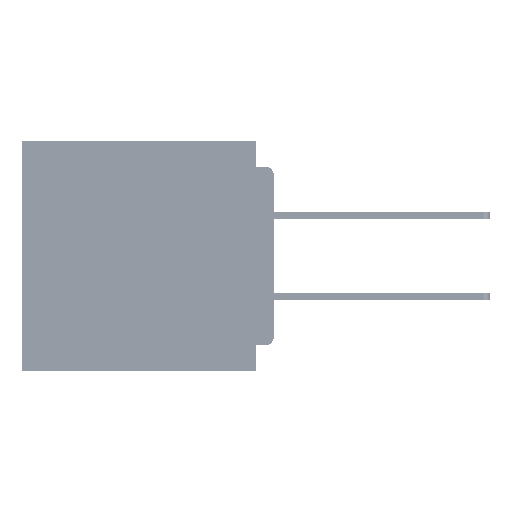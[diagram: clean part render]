
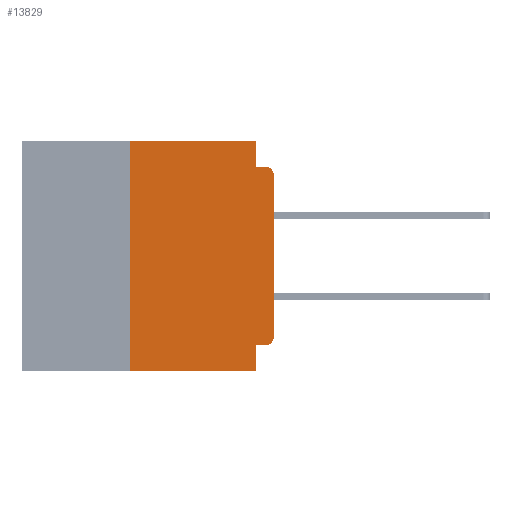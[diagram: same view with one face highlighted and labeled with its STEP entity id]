
A CAD part, left-side view. The second image highlights one B-rep face of the part: STEP entity #13829.
In plain terms, the highlighted planar face has unit normal (-1, 0, 0).
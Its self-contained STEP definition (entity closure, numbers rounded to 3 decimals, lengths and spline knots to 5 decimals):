
#407 = CARTESIAN_POINT ( 'NONE',  ( 0., 0.031, 0. ) ) ;
#1794 = EDGE_CURVE ( 'NONE', #19560, #12595, #44876, .T. ) ;
#2747 = CARTESIAN_POINT ( 'NONE',  ( 0., 0.015, -0.34 ) ) ;
#4199 = CARTESIAN_POINT ( 'NONE',  ( 0., 0.25, -0.4 ) ) ;
#4252 = CARTESIAN_POINT ( 'NONE',  ( 0., 0.015, -0.355 ) ) ;
#5494 = CARTESIAN_POINT ( 'NONE',  ( 0., 0.437, 0. ) ) ;
#5735 = CARTESIAN_POINT ( 'NONE',  ( 0., 0.015, -0.06 ) ) ;
#5874 = VECTOR ( 'NONE', #9253, 39.37008 ) ;
#6515 = CARTESIAN_POINT ( 'NONE',  ( 0., 0., -0.045 ) ) ;
#7438 = EDGE_CURVE ( 'NONE', #57611, #23635, #48891, .T. ) ;
#8135 = DIRECTION ( 'NONE',  ( 0., 0., -1. ) ) ;
#8783 = EDGE_CURVE ( 'NONE', #15629, #69015, #44336, .T. ) ;
#9253 = DIRECTION ( 'NONE',  ( 0., 0., 1. ) ) ;
#9871 = ORIENTED_EDGE ( 'NONE', *, *, #8783, .F. ) ;
#10926 = DIRECTION ( 'NONE',  ( 0., 0., -1. ) ) ;
#11012 = CARTESIAN_POINT ( 'NONE',  ( 0., 0., -0.06 ) ) ;
#11158 = DIRECTION ( 'NONE',  ( 0., 0., -1. ) ) ;
#11940 = DIRECTION ( 'NONE',  ( 0., -1., 0. ) ) ;
#12595 = VERTEX_POINT ( 'NONE', #38211 ) ;
#13058 = VERTEX_POINT ( 'NONE', #36947 ) ;
#13829 = ADVANCED_FACE ( 'NONE', ( #20049 ), #37810, .F. ) ;
#14296 = ORIENTED_EDGE ( 'NONE', *, *, #38138, .T. ) ;
#14543 = ORIENTED_EDGE ( 'NONE', *, *, #32915, .F. ) ;
#15309 = CARTESIAN_POINT ( 'NONE',  ( 0., 0.437, -0.4 ) ) ;
#15629 = VERTEX_POINT ( 'NONE', #18080 ) ;
#15731 = VECTOR ( 'NONE', #47427, 39.37008 ) ;
#16942 = AXIS2_PLACEMENT_3D ( 'NONE', #5735, #43490, #11158 ) ;
#17808 = VECTOR ( 'NONE', #47889, 39.37008 ) ;
#18080 = CARTESIAN_POINT ( 'NONE',  ( 0., 0.031, -0.045 ) ) ;
#18608 = AXIS2_PLACEMENT_3D ( 'NONE', #5494, #43238, #10926 ) ;
#19560 = VERTEX_POINT ( 'NONE', #22905 ) ;
#20049 = FACE_OUTER_BOUND ( 'NONE', #64207, .T. ) ;
#20564 = CARTESIAN_POINT ( 'NONE',  ( 0., 0.437, 0. ) ) ;
#20596 = ORIENTED_EDGE ( 'NONE', *, *, #65454, .F. ) ;
#20742 = DIRECTION ( 'NONE',  ( 0., -1., 0. ) ) ;
#21461 = VECTOR ( 'NONE', #57804, 39.37008 ) ;
#21703 = VECTOR ( 'NONE', #59633, 39.37008 ) ;
#22905 = CARTESIAN_POINT ( 'NONE',  ( 0., 0.031, -0.355 ) ) ;
#23132 = LINE ( 'NONE', #4199, #21461 ) ;
#23635 = VERTEX_POINT ( 'NONE', #11012 ) ;
#24764 = AXIS2_PLACEMENT_3D ( 'NONE', #2747, #40465, #8135 ) ;
#25825 = LINE ( 'NONE', #26003, #65264 ) ;
#26003 = CARTESIAN_POINT ( 'NONE',  ( 0., 0., -0.355 ) ) ;
#26075 = ORIENTED_EDGE ( 'NONE', *, *, #66577, .F. ) ;
#26762 = ORIENTED_EDGE ( 'NONE', *, *, #7438, .T. ) ;
#29517 = EDGE_CURVE ( 'NONE', #23635, #69015, #42485, .T. ) ;
#29912 = VECTOR ( 'NONE', #11940, 39.37008 ) ;
#30033 = LINE ( 'NONE', #20564, #15731 ) ;
#31403 = DIRECTION ( 'NONE',  ( 0., 1., 0. ) ) ;
#32915 = EDGE_CURVE ( 'NONE', #46922, #15629, #50357, .T. ) ;
#35875 = VECTOR ( 'NONE', #20742, 39.37008 ) ;
#36947 = CARTESIAN_POINT ( 'NONE',  ( 0., 0.25, -0.4 ) ) ;
#37810 = PLANE ( 'NONE',  #18608 ) ;
#38124 = ORIENTED_EDGE ( 'NONE', *, *, #44672, .F. ) ;
#38138 = EDGE_CURVE ( 'NONE', #62422, #57611, #43478, .T. ) ;
#38211 = CARTESIAN_POINT ( 'NONE',  ( 0., 0.031, -0.4 ) ) ;
#40136 = CARTESIAN_POINT ( 'NONE',  ( 0., 0.25, 0. ) ) ;
#40465 = DIRECTION ( 'NONE',  ( -1., 0., 0. ) ) ;
#42246 = ORIENTED_EDGE ( 'NONE', *, *, #29517, .T. ) ;
#42485 = CIRCLE ( 'NONE', #16942, 0.015 ) ;
#43238 = DIRECTION ( 'NONE',  ( 1., 0., 0. ) ) ;
#43478 = CIRCLE ( 'NONE', #24764, 0.015 ) ;
#43490 = DIRECTION ( 'NONE',  ( -1., 0., 0. ) ) ;
#44336 = LINE ( 'NONE', #6515, #29912 ) ;
#44672 = EDGE_CURVE ( 'NONE', #49703, #46922, #30033, .T. ) ;
#44876 = LINE ( 'NONE', #48356, #17808 ) ;
#45182 = EDGE_CURVE ( 'NONE', #13058, #12595, #50220, .T. ) ;
#46922 = VERTEX_POINT ( 'NONE', #54579 ) ;
#47427 = DIRECTION ( 'NONE',  ( 0., -1., 0. ) ) ;
#47889 = DIRECTION ( 'NONE',  ( 0., 0., -1. ) ) ;
#48356 = CARTESIAN_POINT ( 'NONE',  ( 0., 0.031, -0.4 ) ) ;
#48891 = LINE ( 'NONE', #62580, #5874 ) ;
#49703 = VERTEX_POINT ( 'NONE', #40136 ) ;
#50220 = LINE ( 'NONE', #15309, #35875 ) ;
#50357 = LINE ( 'NONE', #407, #21703 ) ;
#53339 = CARTESIAN_POINT ( 'NONE',  ( 0., 0., -0.34 ) ) ;
#54579 = CARTESIAN_POINT ( 'NONE',  ( 0., 0.031, 0. ) ) ;
#57611 = VERTEX_POINT ( 'NONE', #53339 ) ;
#57804 = DIRECTION ( 'NONE',  ( 0., 0., 1. ) ) ;
#57962 = CARTESIAN_POINT ( 'NONE',  ( 0., 0.015, -0.045 ) ) ;
#58114 = ORIENTED_EDGE ( 'NONE', *, *, #45182, .T. ) ;
#59633 = DIRECTION ( 'NONE',  ( 0., 0., -1. ) ) ;
#62422 = VERTEX_POINT ( 'NONE', #4252 ) ;
#62580 = CARTESIAN_POINT ( 'NONE',  ( 0., 0., 0. ) ) ;
#64207 = EDGE_LOOP ( 'NONE', ( #26762, #42246, #9871, #14543, #38124, #26075, #58114, #68361, #20596, #14296 ) ) ;
#65264 = VECTOR ( 'NONE', #31403, 39.37008 ) ;
#65454 = EDGE_CURVE ( 'NONE', #62422, #19560, #25825, .T. ) ;
#66577 = EDGE_CURVE ( 'NONE', #13058, #49703, #23132, .T. ) ;
#68361 = ORIENTED_EDGE ( 'NONE', *, *, #1794, .F. ) ;
#69015 = VERTEX_POINT ( 'NONE', #57962 ) ;
